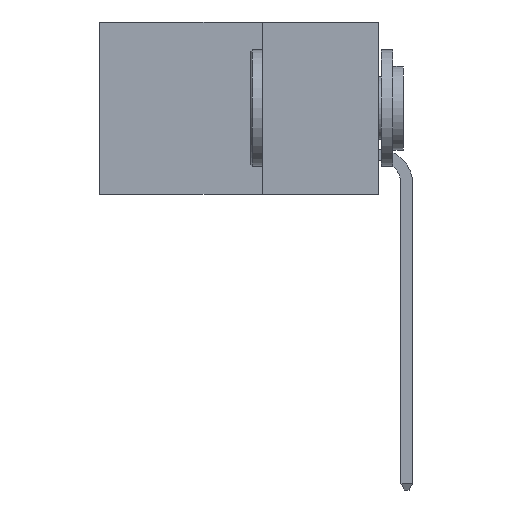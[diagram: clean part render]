
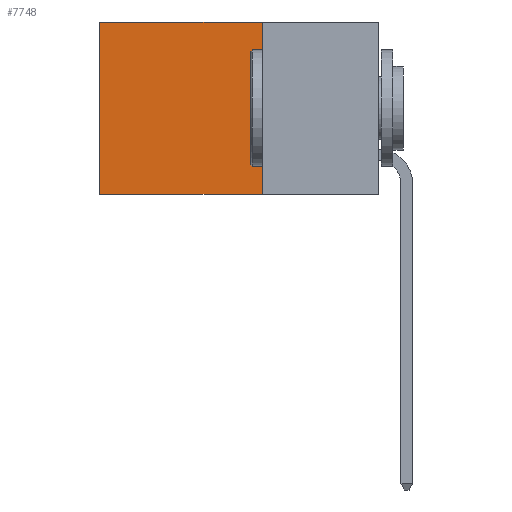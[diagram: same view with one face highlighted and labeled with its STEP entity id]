
A CAD part, left-side view. The second image highlights one B-rep face of the part: STEP entity #7748.
In plain terms, the highlighted planar face has unit normal (-1, 0, 0).
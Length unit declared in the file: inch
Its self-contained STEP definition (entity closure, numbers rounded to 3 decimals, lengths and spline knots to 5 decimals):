
#976 = LINE ( 'NONE', #5317, #10170 ) ;
#2365 = DIRECTION ( 'NONE',  ( 0., 0., -1. ) ) ;
#3113 = VERTEX_POINT ( 'NONE', #12460 ) ;
#3476 = CARTESIAN_POINT ( 'NONE',  ( 0.2615, 0.6, -0.37 ) ) ;
#3682 = LINE ( 'NONE', #12185, #9246 ) ;
#4955 = DIRECTION ( 'NONE',  ( 0., 1., 0. ) ) ;
#4981 = CARTESIAN_POINT ( 'NONE',  ( 0.2615, 0.25, -0.37 ) ) ;
#5317 = CARTESIAN_POINT ( 'NONE',  ( 0.2615, 0.25, 0. ) ) ;
#5801 = VERTEX_POINT ( 'NONE', #3476 ) ;
#6498 = DIRECTION ( 'NONE',  ( 0., 0., -1. ) ) ;
#6567 = CARTESIAN_POINT ( 'NONE',  ( 0.2615, 0.25, -0.37 ) ) ;
#6864 = DIRECTION ( 'NONE',  ( 1., 0., 0. ) ) ;
#7194 = PLANE ( 'NONE',  #24708 ) ;
#7748 = ADVANCED_FACE ( 'NONE', ( #16656 ), #7194, .F. ) ;
#7887 = ORIENTED_EDGE ( 'NONE', *, *, #9155, .F. ) ;
#9117 = VERTEX_POINT ( 'NONE', #12472 ) ;
#9155 = EDGE_CURVE ( 'NONE', #18314, #5801, #3682, .T. ) ;
#9246 = VECTOR ( 'NONE', #12034, 39.37008 ) ;
#9732 = EDGE_CURVE ( 'NONE', #9117, #3113, #976, .T. ) ;
#10170 = VECTOR ( 'NONE', #4955, 39.37008 ) ;
#10189 = EDGE_LOOP ( 'NONE', ( #25170, #7887, #17889, #19284 ) ) ;
#10224 = LINE ( 'NONE', #14938, #19760 ) ;
#12034 = DIRECTION ( 'NONE',  ( 0., 1., 0. ) ) ;
#12185 = CARTESIAN_POINT ( 'NONE',  ( 0.2615, 0.25, -0.37 ) ) ;
#12460 = CARTESIAN_POINT ( 'NONE',  ( 0.2615, 0.6, 0. ) ) ;
#12472 = CARTESIAN_POINT ( 'NONE',  ( 0.2615, 0.25, 0. ) ) ;
#14938 = CARTESIAN_POINT ( 'NONE',  ( 0.2615, 0.6, -0.37 ) ) ;
#16282 = LINE ( 'NONE', #24737, #26205 ) ;
#16656 = FACE_OUTER_BOUND ( 'NONE', #10189, .T. ) ;
#16979 = DIRECTION ( 'NONE',  ( 0., 0., -1. ) ) ;
#17889 = ORIENTED_EDGE ( 'NONE', *, *, #24664, .F. ) ;
#18314 = VERTEX_POINT ( 'NONE', #4981 ) ;
#19284 = ORIENTED_EDGE ( 'NONE', *, *, #9732, .T. ) ;
#19760 = VECTOR ( 'NONE', #16979, 39.37008 ) ;
#24664 = EDGE_CURVE ( 'NONE', #9117, #18314, #16282, .T. ) ;
#24708 = AXIS2_PLACEMENT_3D ( 'NONE', #6567, #6864, #6498 ) ;
#24733 = EDGE_CURVE ( 'NONE', #3113, #5801, #10224, .T. ) ;
#24737 = CARTESIAN_POINT ( 'NONE',  ( 0.2615, 0.25, -0.37 ) ) ;
#25170 = ORIENTED_EDGE ( 'NONE', *, *, #24733, .T. ) ;
#26205 = VECTOR ( 'NONE', #2365, 39.37008 ) ;
